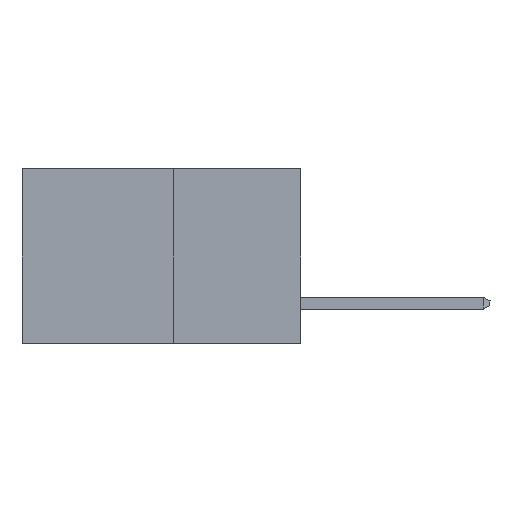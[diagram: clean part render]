
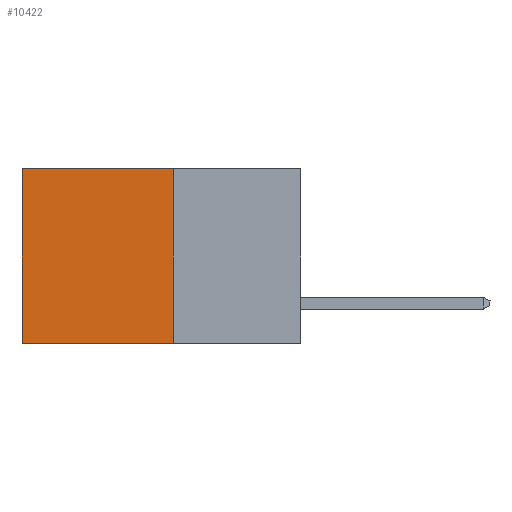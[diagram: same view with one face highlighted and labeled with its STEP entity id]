
A CAD part, left-side view. The second image highlights one B-rep face of the part: STEP entity #10422.
In plain terms, the highlighted planar face has unit normal (-1, 0, 0).
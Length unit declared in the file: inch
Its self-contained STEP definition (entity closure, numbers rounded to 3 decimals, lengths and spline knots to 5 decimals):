
#85 = VERTEX_POINT ( 'NONE', #5868 ) ;
#456 = VERTEX_POINT ( 'NONE', #7368 ) ;
#733 = DIRECTION ( 'NONE',  ( 0., 1., 0. ) ) ;
#785 = EDGE_CURVE ( 'NONE', #456, #85, #12115, .T. ) ;
#852 = AXIS2_PLACEMENT_3D ( 'NONE', #1197, #8049, #2259 ) ;
#1197 = CARTESIAN_POINT ( 'NONE',  ( 0.277, 0.27, -0.37 ) ) ;
#1522 = VERTEX_POINT ( 'NONE', #3532 ) ;
#1575 = DIRECTION ( 'NONE',  ( 0., 1., 0. ) ) ;
#1812 = CARTESIAN_POINT ( 'NONE',  ( 0.277, 0.27, 0. ) ) ;
#2259 = DIRECTION ( 'NONE',  ( 0., 0., -1. ) ) ;
#3227 = PLANE ( 'NONE',  #852 ) ;
#3532 = CARTESIAN_POINT ( 'NONE',  ( 0.277, 0.59, -0.37 ) ) ;
#3900 = EDGE_LOOP ( 'NONE', ( #10112, #11381, #8547, #7016 ) ) ;
#3902 = EDGE_CURVE ( 'NONE', #85, #1522, #6108, .T. ) ;
#3959 = CARTESIAN_POINT ( 'NONE',  ( 0.277, 0.59, 0. ) ) ;
#4589 = CARTESIAN_POINT ( 'NONE',  ( 0.277, 0.27, -0.37 ) ) ;
#5303 = LINE ( 'NONE', #1812, #9508 ) ;
#5868 = CARTESIAN_POINT ( 'NONE',  ( 0.277, 0.27, -0.37 ) ) ;
#6108 = LINE ( 'NONE', #4589, #8225 ) ;
#6690 = CARTESIAN_POINT ( 'NONE',  ( 0.277, 0.59, -0.37 ) ) ;
#7016 = ORIENTED_EDGE ( 'NONE', *, *, #9495, .T. ) ;
#7313 = DIRECTION ( 'NONE',  ( 0., 0., -1. ) ) ;
#7368 = CARTESIAN_POINT ( 'NONE',  ( 0.277, 0.27, 0. ) ) ;
#7571 = CARTESIAN_POINT ( 'NONE',  ( 0.277, 0.27, -0.37 ) ) ;
#7644 = DIRECTION ( 'NONE',  ( 0., 0., -1. ) ) ;
#8049 = DIRECTION ( 'NONE',  ( 1., 0., 0. ) ) ;
#8225 = VECTOR ( 'NONE', #1575, 39.37008 ) ;
#8547 = ORIENTED_EDGE ( 'NONE', *, *, #785, .F. ) ;
#9233 = VECTOR ( 'NONE', #7644, 39.37008 ) ;
#9495 = EDGE_CURVE ( 'NONE', #456, #10926, #5303, .T. ) ;
#9508 = VECTOR ( 'NONE', #733, 39.37008 ) ;
#9844 = VECTOR ( 'NONE', #7313, 39.37008 ) ;
#10112 = ORIENTED_EDGE ( 'NONE', *, *, #10809, .T. ) ;
#10422 = ADVANCED_FACE ( 'NONE', ( #10740 ), #3227, .F. ) ;
#10740 = FACE_OUTER_BOUND ( 'NONE', #3900, .T. ) ;
#10809 = EDGE_CURVE ( 'NONE', #10926, #1522, #11528, .T. ) ;
#10926 = VERTEX_POINT ( 'NONE', #3959 ) ;
#11381 = ORIENTED_EDGE ( 'NONE', *, *, #3902, .F. ) ;
#11528 = LINE ( 'NONE', #6690, #9233 ) ;
#12115 = LINE ( 'NONE', #7571, #9844 ) ;
